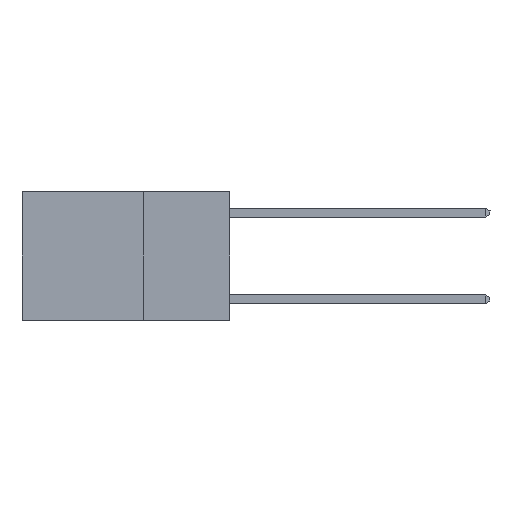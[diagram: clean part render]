
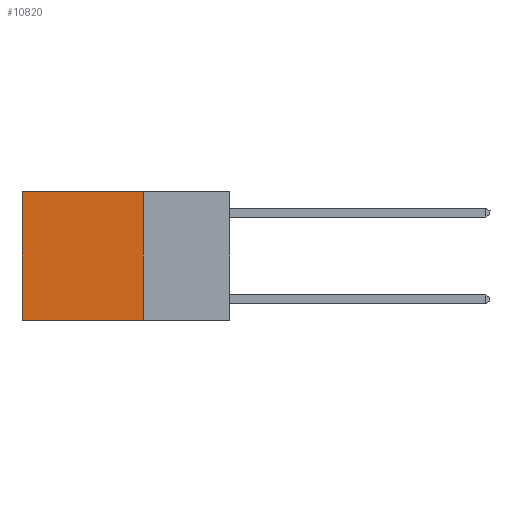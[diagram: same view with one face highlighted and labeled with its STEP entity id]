
A CAD part, left-side view. The second image highlights one B-rep face of the part: STEP entity #10820.
In plain terms, the highlighted planar face has unit normal (-1, 0, 0).
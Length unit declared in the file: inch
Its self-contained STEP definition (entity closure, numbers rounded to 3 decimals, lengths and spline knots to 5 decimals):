
#315 = ORIENTED_EDGE ( 'NONE', *, *, #8156, .T. ) ;
#825 = CARTESIAN_POINT ( 'NONE',  ( 0.2625, 0.25, 0. ) ) ;
#920 = VECTOR ( 'NONE', #3898, 39.37008 ) ;
#2180 = DIRECTION ( 'NONE',  ( 0., 0., -1. ) ) ;
#2521 = CARTESIAN_POINT ( 'NONE',  ( 0.2625, 0.25, 0. ) ) ;
#3898 = DIRECTION ( 'NONE',  ( 0., 1., 0. ) ) ;
#4096 = CARTESIAN_POINT ( 'NONE',  ( 0.2625, 0.25, -0.37 ) ) ;
#4164 = CARTESIAN_POINT ( 'NONE',  ( 0.2625, 0.25, 0. ) ) ;
#4191 = VERTEX_POINT ( 'NONE', #8892 ) ;
#4328 = EDGE_CURVE ( 'NONE', #7084, #12181, #11512, .T. ) ;
#5182 = LINE ( 'NONE', #12571, #16006 ) ;
#7084 = VERTEX_POINT ( 'NONE', #4164 ) ;
#7120 = FACE_OUTER_BOUND ( 'NONE', #16916, .T. ) ;
#7577 = CARTESIAN_POINT ( 'NONE',  ( 0.2625, 0.6, 0. ) ) ;
#7833 = VECTOR ( 'NONE', #8883, 39.37008 ) ;
#8060 = EDGE_CURVE ( 'NONE', #7084, #11114, #9439, .T. ) ;
#8156 = EDGE_CURVE ( 'NONE', #12181, #4191, #11212, .T. ) ;
#8883 = DIRECTION ( 'NONE',  ( 0., 0., -1. ) ) ;
#8892 = CARTESIAN_POINT ( 'NONE',  ( 0.2625, 0.6, -0.37 ) ) ;
#9050 = VECTOR ( 'NONE', #11264, 39.37008 ) ;
#9439 = LINE ( 'NONE', #9958, #9050 ) ;
#9958 = CARTESIAN_POINT ( 'NONE',  ( 0.2625, 0.25, 0. ) ) ;
#10157 = DIRECTION ( 'NONE',  ( 1., 0., 0. ) ) ;
#10820 = ADVANCED_FACE ( 'NONE', ( #7120 ), #11393, .F. ) ;
#10954 = ORIENTED_EDGE ( 'NONE', *, *, #14619, .F. ) ;
#11114 = VERTEX_POINT ( 'NONE', #4096 ) ;
#11212 = LINE ( 'NONE', #7577, #7833 ) ;
#11264 = DIRECTION ( 'NONE',  ( 0., 0., -1. ) ) ;
#11393 = PLANE ( 'NONE',  #15525 ) ;
#11512 = LINE ( 'NONE', #2521, #920 ) ;
#11813 = ORIENTED_EDGE ( 'NONE', *, *, #8060, .F. ) ;
#12013 = ORIENTED_EDGE ( 'NONE', *, *, #4328, .T. ) ;
#12181 = VERTEX_POINT ( 'NONE', #14316 ) ;
#12571 = CARTESIAN_POINT ( 'NONE',  ( 0.2625, 0.25, -0.37 ) ) ;
#14316 = CARTESIAN_POINT ( 'NONE',  ( 0.2625, 0.6, 0. ) ) ;
#14619 = EDGE_CURVE ( 'NONE', #11114, #4191, #5182, .T. ) ;
#15525 = AXIS2_PLACEMENT_3D ( 'NONE', #825, #10157, #2180 ) ;
#16006 = VECTOR ( 'NONE', #16423, 39.37008 ) ;
#16423 = DIRECTION ( 'NONE',  ( 0., 1., 0. ) ) ;
#16916 = EDGE_LOOP ( 'NONE', ( #315, #10954, #11813, #12013 ) ) ;
